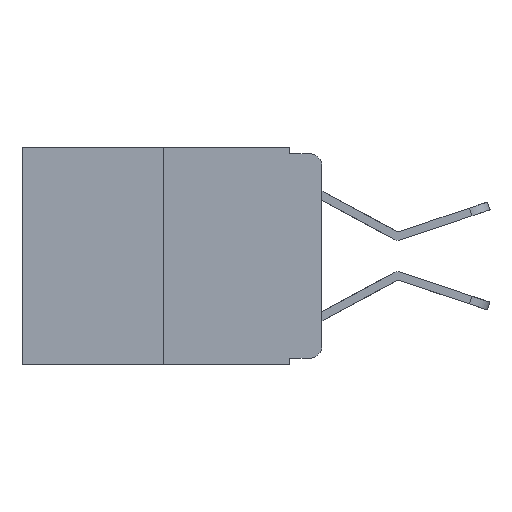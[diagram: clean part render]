
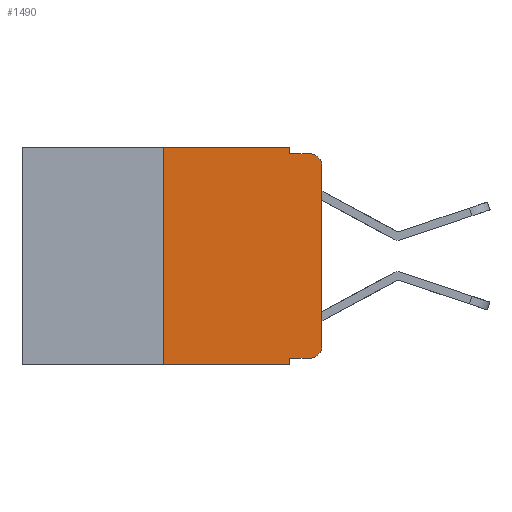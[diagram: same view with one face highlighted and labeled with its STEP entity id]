
A CAD part, left-side view. The second image highlights one B-rep face of the part: STEP entity #1490.
In plain terms, the highlighted planar face has unit normal (-1, 0, 0).
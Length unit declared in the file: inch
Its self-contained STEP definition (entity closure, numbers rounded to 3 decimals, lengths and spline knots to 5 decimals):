
#29 = VERTEX_POINT ( 'NONE', #14055 ) ;
#350 = LINE ( 'NONE', #11090, #20947 ) ;
#415 = EDGE_CURVE ( 'NONE', #29, #14120, #12753, .T. ) ;
#759 = VERTEX_POINT ( 'NONE', #8772 ) ;
#921 = CARTESIAN_POINT ( 'NONE',  ( 0., 0.051, -0.01 ) ) ;
#1366 = VERTEX_POINT ( 'NONE', #23308 ) ;
#1490 = ADVANCED_FACE ( 'NONE', ( #17263 ), #20610, .F. ) ;
#1564 = ORIENTED_EDGE ( 'NONE', *, *, #4615, .T. ) ;
#3231 = EDGE_CURVE ( 'NONE', #14120, #11885, #10520, .T. ) ;
#3276 = DIRECTION ( 'NONE',  ( 0., 0., 1. ) ) ;
#3987 = CARTESIAN_POINT ( 'NONE',  ( 0., 0., 0. ) ) ;
#4166 = CARTESIAN_POINT ( 'NONE',  ( 0., 0.051, 0. ) ) ;
#4539 = ORIENTED_EDGE ( 'NONE', *, *, #5989, .T. ) ;
#4615 = EDGE_CURVE ( 'NONE', #15490, #11885, #17143, .T. ) ;
#5562 = CARTESIAN_POINT ( 'NONE',  ( 0., 0.02, -0.313 ) ) ;
#5910 = EDGE_CURVE ( 'NONE', #1366, #24229, #14353, .T. ) ;
#5989 = EDGE_CURVE ( 'NONE', #759, #15490, #12522, .T. ) ;
#6426 = VECTOR ( 'NONE', #3276, 39.37008 ) ;
#6445 = LINE ( 'NONE', #4166, #7088 ) ;
#7088 = VECTOR ( 'NONE', #19992, 39.37008 ) ;
#7089 = ORIENTED_EDGE ( 'NONE', *, *, #23540, .F. ) ;
#7180 = VECTOR ( 'NONE', #10198, 39.37008 ) ;
#7186 = CARTESIAN_POINT ( 'NONE',  ( 0., 0.051, -0.333 ) ) ;
#7434 = VECTOR ( 'NONE', #9630, 39.37008 ) ;
#7629 = CARTESIAN_POINT ( 'NONE',  ( 0., 0.02, -0.03 ) ) ;
#7656 = DIRECTION ( 'NONE',  ( 0., 0., -1. ) ) ;
#8772 = CARTESIAN_POINT ( 'NONE',  ( 0., 0., -0.313 ) ) ;
#9452 = CARTESIAN_POINT ( 'NONE',  ( 0., 0.051, 0. ) ) ;
#9630 = DIRECTION ( 'NONE',  ( 0., 0., -1. ) ) ;
#9702 = DIRECTION ( 'NONE',  ( 0., 0., -1. ) ) ;
#9783 = LINE ( 'NONE', #10048, #10419 ) ;
#9930 = CARTESIAN_POINT ( 'NONE',  ( 0., 0.473, -0.343 ) ) ;
#10048 = CARTESIAN_POINT ( 'NONE',  ( 0., 0.051, -0.333 ) ) ;
#10198 = DIRECTION ( 'NONE',  ( 0., 0., 1. ) ) ;
#10419 = VECTOR ( 'NONE', #13857, 39.37008 ) ;
#10520 = LINE ( 'NONE', #921, #19600 ) ;
#10534 = VERTEX_POINT ( 'NONE', #24326 ) ;
#11005 = DIRECTION ( 'NONE',  ( 1., 0., 0. ) ) ;
#11025 = DIRECTION ( 'NONE',  ( 0., 0., -1. ) ) ;
#11090 = CARTESIAN_POINT ( 'NONE',  ( 0., 0.473, 0. ) ) ;
#11885 = VERTEX_POINT ( 'NONE', #15048 ) ;
#12522 = LINE ( 'NONE', #3987, #7180 ) ;
#12753 = LINE ( 'NONE', #9452, #7434 ) ;
#12864 = AXIS2_PLACEMENT_3D ( 'NONE', #14540, #11005, #11025 ) ;
#13047 = DIRECTION ( 'NONE',  ( 0., -1., 0. ) ) ;
#13641 = LINE ( 'NONE', #19169, #6426 ) ;
#13654 = CARTESIAN_POINT ( 'NONE',  ( 0., 0.25, 0. ) ) ;
#13857 = DIRECTION ( 'NONE',  ( 0., -1., 0. ) ) ;
#14055 = CARTESIAN_POINT ( 'NONE',  ( 0., 0.051, 0. ) ) ;
#14120 = VERTEX_POINT ( 'NONE', #14934 ) ;
#14290 = CARTESIAN_POINT ( 'NONE',  ( 0., 0., -0.03 ) ) ;
#14311 = VERTEX_POINT ( 'NONE', #13654 ) ;
#14353 = LINE ( 'NONE', #9930, #23973 ) ;
#14540 = CARTESIAN_POINT ( 'NONE',  ( 0., 0.473, 0. ) ) ;
#14557 = AXIS2_PLACEMENT_3D ( 'NONE', #7629, #21285, #9702 ) ;
#14638 = EDGE_CURVE ( 'NONE', #14311, #29, #350, .T. ) ;
#14934 = CARTESIAN_POINT ( 'NONE',  ( 0., 0.051, -0.01 ) ) ;
#15048 = CARTESIAN_POINT ( 'NONE',  ( 0., 0.02, -0.01 ) ) ;
#15490 = VERTEX_POINT ( 'NONE', #14290 ) ;
#16075 = ORIENTED_EDGE ( 'NONE', *, *, #20967, .T. ) ;
#16886 = CIRCLE ( 'NONE', #24241, 0.02 ) ;
#16990 = DIRECTION ( 'NONE',  ( 0., -1., 0. ) ) ;
#17143 = CIRCLE ( 'NONE', #14557, 0.02 ) ;
#17263 = FACE_OUTER_BOUND ( 'NONE', #22134, .T. ) ;
#17615 = ORIENTED_EDGE ( 'NONE', *, *, #18409, .T. ) ;
#18409 = EDGE_CURVE ( 'NONE', #10534, #759, #16886, .T. ) ;
#19169 = CARTESIAN_POINT ( 'NONE',  ( 0., 0.25, 0. ) ) ;
#19407 = DIRECTION ( 'NONE',  ( -1., 0., 0. ) ) ;
#19600 = VECTOR ( 'NONE', #16990, 39.37008 ) ;
#19705 = ORIENTED_EDGE ( 'NONE', *, *, #5910, .T. ) ;
#19992 = DIRECTION ( 'NONE',  ( 0., 0., -1. ) ) ;
#20219 = VERTEX_POINT ( 'NONE', #7186 ) ;
#20610 = PLANE ( 'NONE',  #12864 ) ;
#20889 = ORIENTED_EDGE ( 'NONE', *, *, #3231, .F. ) ;
#20947 = VECTOR ( 'NONE', #13047, 39.37008 ) ;
#20967 = EDGE_CURVE ( 'NONE', #20219, #10534, #9783, .T. ) ;
#21148 = ORIENTED_EDGE ( 'NONE', *, *, #14638, .F. ) ;
#21285 = DIRECTION ( 'NONE',  ( -1., 0., 0. ) ) ;
#21492 = ORIENTED_EDGE ( 'NONE', *, *, #24792, .F. ) ;
#22134 = EDGE_LOOP ( 'NONE', ( #4539, #1564, #20889, #24413, #21148, #21492, #19705, #7089, #16075, #17615 ) ) ;
#23308 = CARTESIAN_POINT ( 'NONE',  ( 0., 0.25, -0.343 ) ) ;
#23410 = DIRECTION ( 'NONE',  ( 0., -1., 0. ) ) ;
#23540 = EDGE_CURVE ( 'NONE', #20219, #24229, #6445, .T. ) ;
#23973 = VECTOR ( 'NONE', #23410, 39.37008 ) ;
#24229 = VERTEX_POINT ( 'NONE', #25103 ) ;
#24241 = AXIS2_PLACEMENT_3D ( 'NONE', #5562, #19407, #7656 ) ;
#24326 = CARTESIAN_POINT ( 'NONE',  ( 0., 0.02, -0.333 ) ) ;
#24413 = ORIENTED_EDGE ( 'NONE', *, *, #415, .F. ) ;
#24792 = EDGE_CURVE ( 'NONE', #1366, #14311, #13641, .T. ) ;
#25103 = CARTESIAN_POINT ( 'NONE',  ( 0., 0.051, -0.343 ) ) ;
